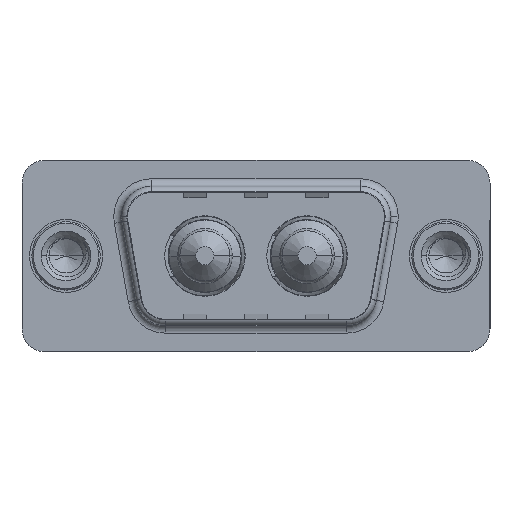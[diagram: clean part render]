
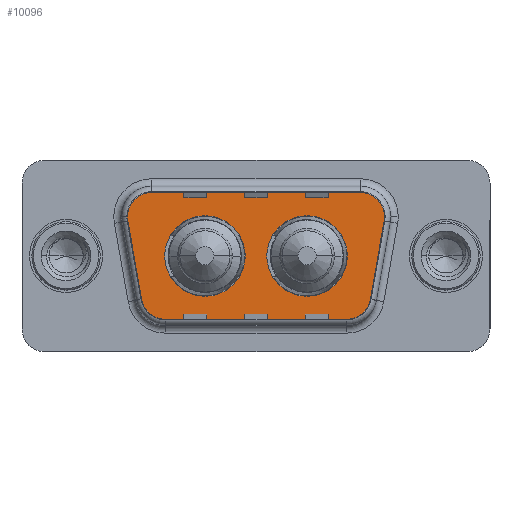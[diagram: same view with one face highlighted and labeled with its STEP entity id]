
A CAD part, top view. The second image highlights one B-rep face of the part: STEP entity #10096.
In plain terms, the highlighted planar face has unit normal (0, 0, 1).
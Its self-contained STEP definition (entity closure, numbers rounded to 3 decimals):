
#57 = VERTEX_POINT ( 'NONE', #4843 ) ;
#73 = CIRCLE ( 'NONE', #2746, 2. ) ;
#253 = DIRECTION ( 'NONE',  ( 0., 0., 1. ) ) ;
#256 = CIRCLE ( 'NONE', #7858, 2. ) ;
#257 = ORIENTED_EDGE ( 'NONE', *, *, #689, .T. ) ;
#277 = AXIS2_PLACEMENT_3D ( 'NONE', #11885, #842, #6403 ) ;
#288 = CARTESIAN_POINT ( 'NONE',  ( 15.86, 0., 0. ) ) ;
#385 = DIRECTION ( 'NONE',  ( 1., 0., 0. ) ) ;
#400 = CIRCLE ( 'NONE', #9893, 2.65 ) ;
#504 = CARTESIAN_POINT ( 'NONE',  ( 3.466, 2.553, 0. ) ) ;
#638 = CARTESIAN_POINT ( 'NONE',  ( 6.49, 0., 0. ) ) ;
#680 = CARTESIAN_POINT ( 'NONE',  ( 18.541, -4.9, 0. ) ) ;
#689 = EDGE_CURVE ( 'NONE', #2791, #4216, #3997, .T. ) ;
#842 = DIRECTION ( 'NONE',  ( 0., 0., 1. ) ) ;
#931 = FACE_OUTER_BOUND ( 'NONE', #10666, .T. ) ;
#1238 = VERTEX_POINT ( 'NONE', #6708 ) ;
#1518 = ORIENTED_EDGE ( 'NONE', *, *, #4053, .F. ) ;
#1568 = AXIS2_PLACEMENT_3D ( 'NONE', #288, #253, #4766 ) ;
#1752 = CARTESIAN_POINT ( 'NONE',  ( 4.489, -3.247, 0. ) ) ;
#1764 = DIRECTION ( 'NONE',  ( 0.174, 0.985, 0. ) ) ;
#1882 = EDGE_CURVE ( 'NONE', #3055, #5344, #3980, .T. ) ;
#1997 = EDGE_CURVE ( 'NONE', #5637, #3075, #3397, .T. ) ;
#2107 = LINE ( 'NONE', #3246, #9143 ) ;
#2415 = VERTEX_POINT ( 'NONE', #1752 ) ;
#2694 = ORIENTED_EDGE ( 'NONE', *, *, #3946, .T. ) ;
#2746 = AXIS2_PLACEMENT_3D ( 'NONE', #10160, #4683, #11090 ) ;
#2791 = VERTEX_POINT ( 'NONE', #4671 ) ;
#2963 = CARTESIAN_POINT ( 'NONE',  ( 20.511, -3.247, 0. ) ) ;
#3000 = VERTEX_POINT ( 'NONE', #10568 ) ;
#3015 = CARTESIAN_POINT ( 'NONE',  ( 9.14, 0., 0. ) ) ;
#3043 = CARTESIAN_POINT ( 'NONE',  ( 6.459, -4.9, 0. ) ) ;
#3055 = VERTEX_POINT ( 'NONE', #638 ) ;
#3075 = VERTEX_POINT ( 'NONE', #8159 ) ;
#3246 = CARTESIAN_POINT ( 'NONE',  ( 5.436, 4.9, 0. ) ) ;
#3377 = DIRECTION ( 'NONE',  ( 0., 0., 1. ) ) ;
#3397 = CIRCLE ( 'NONE', #1568, 2.65 ) ;
#3412 = ORIENTED_EDGE ( 'NONE', *, *, #7865, .T. ) ;
#3490 = DIRECTION ( 'NONE',  ( 0., 0., 1. ) ) ;
#3632 = VERTEX_POINT ( 'NONE', #2963 ) ;
#3720 = ORIENTED_EDGE ( 'NONE', *, *, #9292, .T. ) ;
#3777 = DIRECTION ( 'NONE',  ( 0., 0., 1. ) ) ;
#3945 = DIRECTION ( 'NONE',  ( 1., 0., 0. ) ) ;
#3946 = EDGE_CURVE ( 'NONE', #2415, #4821, #6460, .T. ) ;
#3980 = CIRCLE ( 'NONE', #6776, 2.65 ) ;
#3997 = CIRCLE ( 'NONE', #6449, 2. ) ;
#4051 = DIRECTION ( 'NONE',  ( 1., 0., 0. ) ) ;
#4053 = EDGE_CURVE ( 'NONE', #3075, #5637, #400, .T. ) ;
#4098 = DIRECTION ( 'NONE',  ( 0., 0., 1. ) ) ;
#4105 = ORIENTED_EDGE ( 'NONE', *, *, #11196, .T. ) ;
#4216 = VERTEX_POINT ( 'NONE', #4868 ) ;
#4407 = EDGE_CURVE ( 'NONE', #5106, #3632, #256, .T. ) ;
#4434 = ORIENTED_EDGE ( 'NONE', *, *, #11034, .T. ) ;
#4496 = VECTOR ( 'NONE', #1764, 1000. ) ;
#4671 = CARTESIAN_POINT ( 'NONE',  ( 5.436, 4.9, 0. ) ) ;
#4683 = DIRECTION ( 'NONE',  ( 0., 0., 1. ) ) ;
#4766 = DIRECTION ( 'NONE',  ( 1., 0., 0. ) ) ;
#4821 = VERTEX_POINT ( 'NONE', #3043 ) ;
#4843 = CARTESIAN_POINT ( 'NONE',  ( 21.534, 2.553, 0. ) ) ;
#4866 = CARTESIAN_POINT ( 'NONE',  ( 9.14, 0., 0. ) ) ;
#4868 = CARTESIAN_POINT ( 'NONE',  ( 3.466, 2.553, 0. ) ) ;
#4946 = EDGE_CURVE ( 'NONE', #1238, #2791, #2107, .T. ) ;
#4956 = CIRCLE ( 'NONE', #10680, 2. ) ;
#5025 = DIRECTION ( 'NONE',  ( -1., 0., 0. ) ) ;
#5045 = DIRECTION ( 'NONE',  ( -1., 0., 0. ) ) ;
#5046 = DIRECTION ( 'NONE',  ( 0., 0., 1. ) ) ;
#5061 = CARTESIAN_POINT ( 'NONE',  ( 6.459, -2.9, 0. ) ) ;
#5106 = VERTEX_POINT ( 'NONE', #680 ) ;
#5344 = VERTEX_POINT ( 'NONE', #5681 ) ;
#5610 = AXIS2_PLACEMENT_3D ( 'NONE', #5061, #5046, #5025 ) ;
#5637 = VERTEX_POINT ( 'NONE', #9949 ) ;
#5681 = CARTESIAN_POINT ( 'NONE',  ( 11.79, 0., 0. ) ) ;
#5875 = DIRECTION ( 'NONE',  ( 0., 0., 1. ) ) ;
#6047 = EDGE_CURVE ( 'NONE', #5344, #3055, #11165, .T. ) ;
#6403 = DIRECTION ( 'NONE',  ( 1., 0., 0. ) ) ;
#6449 = AXIS2_PLACEMENT_3D ( 'NONE', #10329, #5875, #385 ) ;
#6460 = CIRCLE ( 'NONE', #5610, 2. ) ;
#6694 = LINE ( 'NONE', #11437, #11269 ) ;
#6708 = CARTESIAN_POINT ( 'NONE',  ( 19.564, 4.9, 0. ) ) ;
#6776 = AXIS2_PLACEMENT_3D ( 'NONE', #4866, #4098, #4051 ) ;
#7108 = EDGE_LOOP ( 'NONE', ( #1518, #11530 ) ) ;
#7858 = AXIS2_PLACEMENT_3D ( 'NONE', #8855, #3377, #9765 ) ;
#7865 = EDGE_CURVE ( 'NONE', #3632, #57, #10232, .T. ) ;
#8028 = ORIENTED_EDGE ( 'NONE', *, *, #1882, .F. ) ;
#8159 = CARTESIAN_POINT ( 'NONE',  ( 18.51, 0., 0. ) ) ;
#8270 = ORIENTED_EDGE ( 'NONE', *, *, #4946, .T. ) ;
#8346 = VECTOR ( 'NONE', #8781, 1000. ) ;
#8479 = ORIENTED_EDGE ( 'NONE', *, *, #10165, .T. ) ;
#8669 = DIRECTION ( 'NONE',  ( 1., 0., 0. ) ) ;
#8781 = DIRECTION ( 'NONE',  ( 0.174, -0.985, 0. ) ) ;
#8855 = CARTESIAN_POINT ( 'NONE',  ( 18.541, -2.9, 0. ) ) ;
#8983 = CARTESIAN_POINT ( 'NONE',  ( 19.564, 2.9, 0. ) ) ;
#9143 = VECTOR ( 'NONE', #5045, 1000. ) ;
#9274 = CARTESIAN_POINT ( 'NONE',  ( 15.86, 0., 0. ) ) ;
#9292 = EDGE_CURVE ( 'NONE', #4216, #2415, #10773, .T. ) ;
#9419 = DIRECTION ( 'NONE',  ( 0., 0., 1. ) ) ;
#9765 = DIRECTION ( 'NONE',  ( 1., 0., 0. ) ) ;
#9885 = DIRECTION ( 'NONE',  ( -1., 0., 0. ) ) ;
#9893 = AXIS2_PLACEMENT_3D ( 'NONE', #9274, #3777, #10182 ) ;
#9933 = ORIENTED_EDGE ( 'NONE', *, *, #6047, .F. ) ;
#9949 = CARTESIAN_POINT ( 'NONE',  ( 13.21, 0., 0. ) ) ;
#10096 = ADVANCED_FACE ( 'NONE', ( #10711, #10420, #931 ), #10975, .T. ) ;
#10160 = CARTESIAN_POINT ( 'NONE',  ( 19.564, 2.9, 0. ) ) ;
#10165 = EDGE_CURVE ( 'NONE', #3000, #1238, #73, .T. ) ;
#10182 = DIRECTION ( 'NONE',  ( 1., 0., 0. ) ) ;
#10232 = LINE ( 'NONE', #11851, #4496 ) ;
#10329 = CARTESIAN_POINT ( 'NONE',  ( 5.436, 2.9, 0. ) ) ;
#10420 = FACE_BOUND ( 'NONE', #11122, .T. ) ;
#10541 = ORIENTED_EDGE ( 'NONE', *, *, #4407, .T. ) ;
#10568 = CARTESIAN_POINT ( 'NONE',  ( 21.564, 2.9, 0. ) ) ;
#10666 = EDGE_LOOP ( 'NONE', ( #10541, #3412, #4105, #8479, #8270, #257, #3720, #2694, #4434 ) ) ;
#10680 = AXIS2_PLACEMENT_3D ( 'NONE', #8983, #3490, #9885 ) ;
#10711 = FACE_BOUND ( 'NONE', #7108, .T. ) ;
#10773 = LINE ( 'NONE', #504, #8346 ) ;
#10975 = PLANE ( 'NONE',  #277 ) ;
#11034 = EDGE_CURVE ( 'NONE', #4821, #5106, #6694, .T. ) ;
#11053 = AXIS2_PLACEMENT_3D ( 'NONE', #3015, #9419, #3945 ) ;
#11090 = DIRECTION ( 'NONE',  ( -1., 0., 0. ) ) ;
#11122 = EDGE_LOOP ( 'NONE', ( #9933, #8028 ) ) ;
#11165 = CIRCLE ( 'NONE', #11053, 2.65 ) ;
#11196 = EDGE_CURVE ( 'NONE', #57, #3000, #4956, .T. ) ;
#11269 = VECTOR ( 'NONE', #8669, 1000. ) ;
#11437 = CARTESIAN_POINT ( 'NONE',  ( 6.459, -4.9, 0. ) ) ;
#11530 = ORIENTED_EDGE ( 'NONE', *, *, #1997, .F. ) ;
#11851 = CARTESIAN_POINT ( 'NONE',  ( 21.534, 2.553, 0. ) ) ;
#11885 = CARTESIAN_POINT ( 'NONE',  ( 18.541, -2.9, 0. ) ) ;
